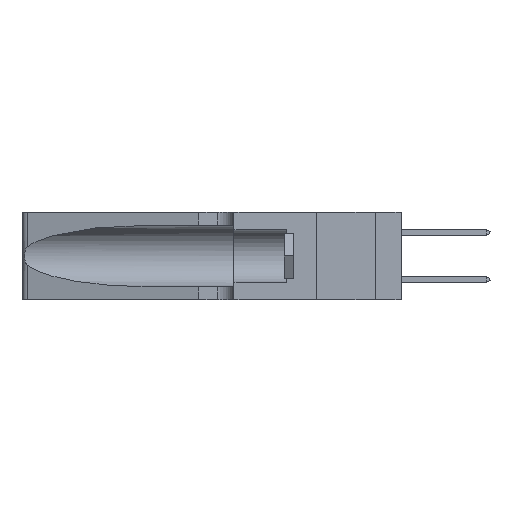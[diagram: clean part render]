
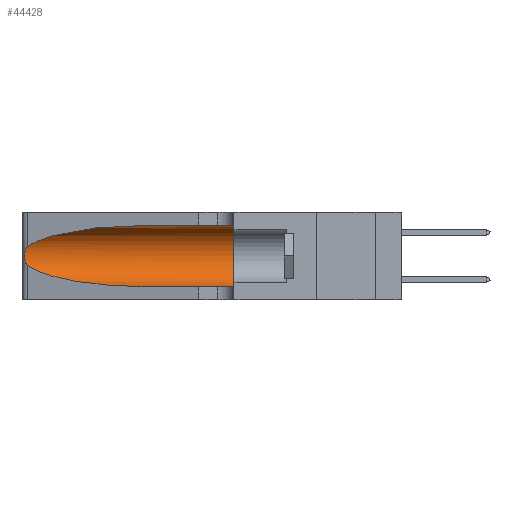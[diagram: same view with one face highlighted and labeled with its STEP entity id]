
A CAD part, left-side view. The second image highlights one B-rep face of the part: STEP entity #44428.
In plain terms, the highlighted cylindrical face has radius 3.308 mm (diameter 6.617 mm), a partial arc.
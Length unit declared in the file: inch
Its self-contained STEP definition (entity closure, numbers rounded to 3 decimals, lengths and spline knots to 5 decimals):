
#996 = CARTESIAN_POINT ( 'NONE',  ( 0.25487, 1.22718, 0.14631 ) ) ;
#1841 = VERTEX_POINT ( 'NONE', #12380 ) ;
#2195 = EDGE_CURVE ( 'NONE', #1841, #40838, #9917, .T. ) ;
#2207 = CARTESIAN_POINT ( 'NONE',  ( 0.25487, 1.22718, 0.22369 ) ) ;
#2439 = DIRECTION ( 'NONE',  ( 0., -1., 0. ) ) ;
#2642 = EDGE_CURVE ( 'NONE', #31339, #1841, #34223, .T. ) ;
#3109 = CARTESIAN_POINT ( 'NONE',  ( 0.1305, 1.61858, 0.31525 ) ) ;
#4090 = CARTESIAN_POINT ( 'NONE',  ( 0.1305, 0.35, 0.185 ) ) ;
#4380 = CARTESIAN_POINT ( 'NONE',  ( 0.25787, 1.23484, 0.2124 ) ) ;
#7574 = CARTESIAN_POINT ( 'NONE',  ( 0.26018, 1.23835, 0.19895 ) ) ;
#9135 = EDGE_CURVE ( 'NONE', #31339, #39985, #35731, .T. ) ;
#9268 = CARTESIAN_POINT ( 'NONE',  ( 0.1305, 1.61858, 0.05475 ) ) ;
#9917 = CIRCLE ( 'NONE', #42887, 0.13025 ) ;
#10337 = ORIENTED_EDGE ( 'NONE', *, *, #40380, .T. ) ;
#11255 = DIRECTION ( 'NONE',  ( 0., 1., 0. ) ) ;
#11530 = FACE_OUTER_BOUND ( 'NONE', #39396, .T. ) ;
#11571 = CARTESIAN_POINT ( 'NONE',  ( 0.25639, 1.23186, 0.15144 ) ) ;
#11637 = VERTEX_POINT ( 'NONE', #42432 ) ;
#12380 = CARTESIAN_POINT ( 'NONE',  ( 0.1305, 0.35, 0.31525 ) ) ;
#13915 = DIRECTION ( 'NONE',  ( 0., 0., -1. ) ) ;
#14069 = VECTOR ( 'NONE', #2439, 39.37008 ) ;
#14387 = CYLINDRICAL_SURFACE ( 'NONE', #37112, 0.13025 ) ;
#14938 = CARTESIAN_POINT ( 'NONE',  ( 0.25487, 1.22718, 0.22369 ) ) ;
#15084 = CARTESIAN_POINT ( 'NONE',  ( 0.25789, 1.23486, 0.15765 ) ) ;
#16788 = CARTESIAN_POINT ( 'NONE',  ( 0.18966, 0.96281, 0.05475 ) ) ;
#17612 = DIRECTION ( 'NONE',  ( 0., -1., 0. ) ) ;
#18283 = CARTESIAN_POINT ( 'NONE',  ( 0.18966, 0.96281, 0.31525 ) ) ;
#18475 = CARTESIAN_POINT ( 'NONE',  ( 0.26075, 1.23896, 0.178 ) ) ;
#18594 = ORIENTED_EDGE ( 'NONE', *, *, #41261, .T. ) ;
#19185 = EDGE_CURVE ( 'NONE', #11637, #39734, #34885, .T. ) ;
#20119 = ORIENTED_EDGE ( 'NONE', *, *, #2642, .F. ) ;
#22096 = CARTESIAN_POINT ( 'NONE',  ( 0.25555, 1.22993, 0.14849 ) ) ;
#22246 = CARTESIAN_POINT ( 'NONE',  ( 0.25639, 1.23184, 0.21858 ) ) ;
#22397 = CARTESIAN_POINT ( 'NONE',  ( 0.25555, 1.22994, 0.2215 ) ) ;
#22699 = CARTESIAN_POINT ( 'NONE',  ( 0.26075, 1.23896, 0.19203 ) ) ;
#23720 = LINE ( 'NONE', #9268, #14069 ) ;
#25239 = CARTESIAN_POINT ( 'NONE',  ( 0.1305, 0.72297, 0.31525 ) ) ;
#25550 = CARTESIAN_POINT ( 'NONE',  ( 0.25487, 1.22718, 0.22369 ) ) ;
#26036 = CARTESIAN_POINT ( 'NONE',  ( 0.25487, 1.22718, 0.14631 ) ) ;
#26040 = DIRECTION ( 'NONE',  ( 0., 0., 1. ) ) ;
#26438 = CARTESIAN_POINT ( 'NONE',  ( 0.2373, 1.15595, 0.08982 ) ) ;
#28228 = ORIENTED_EDGE ( 'NONE', *, *, #2195, .F. ) ;
#30805 = CARTESIAN_POINT ( 'NONE',  ( 0.1305, 0.72297, 0.05475 ) ) ;
#31339 = VERTEX_POINT ( 'NONE', #35454 ) ;
#31789 = CARTESIAN_POINT ( 'NONE',  ( 0.1305, 0.35, 0.05475 ) ) ;
#33256 = CARTESIAN_POINT ( 'NONE',  ( 0.26017, 1.23833, 0.17102 ) ) ;
#34223 = LINE ( 'NONE', #3109, #42796 ) ;
#34885 =( BOUNDED_CURVE ( )  B_SPLINE_CURVE ( 3, ( #996, #26438, #16788, #30805 ),
 .UNSPECIFIED., .F., .T. ) 
 B_SPLINE_CURVE_WITH_KNOTS ( ( 4, 4 ),
 ( 3.44316, 4.71239 ),
 .UNSPECIFIED. ) 
 CURVE ( )  GEOMETRIC_REPRESENTATION_ITEM ( )  RATIONAL_B_SPLINE_CURVE ( ( 1., 0.87, 0.87, 1. ) ) 
 REPRESENTATION_ITEM ( '' )  );
#35209 = ORIENTED_EDGE ( 'NONE', *, *, #19185, .T. ) ;
#35454 = CARTESIAN_POINT ( 'NONE',  ( 0.1305, 0.72297, 0.31525 ) ) ;
#35731 =( BOUNDED_CURVE ( )  B_SPLINE_CURVE ( 3, ( #25239, #18283, #43603, #25550 ),
 .UNSPECIFIED., .F., .F. ) 
 B_SPLINE_CURVE_WITH_KNOTS ( ( 4, 4 ),
 ( 1.5708, 2.84003 ),
 .UNSPECIFIED. ) 
 CURVE ( )  GEOMETRIC_REPRESENTATION_ITEM ( )  RATIONAL_B_SPLINE_CURVE ( ( 1., 0.87, 0.87, 1. ) ) 
 REPRESENTATION_ITEM ( '' )  );
#37112 = AXIS2_PLACEMENT_3D ( 'NONE', #42608, #46564, #13915 ) ;
#39396 = EDGE_LOOP ( 'NONE', ( #39607, #10337, #35209, #18594, #28228, #20119 ) ) ;
#39607 = ORIENTED_EDGE ( 'NONE', *, *, #9135, .T. ) ;
#39734 = VERTEX_POINT ( 'NONE', #44288 ) ;
#39985 = VERTEX_POINT ( 'NONE', #2207 ) ;
#40263 = CARTESIAN_POINT ( 'NONE',  ( 0.25854, 1.2359, 0.20912 ) ) ;
#40380 = EDGE_CURVE ( 'NONE', #39985, #11637, #42755, .T. ) ;
#40838 = VERTEX_POINT ( 'NONE', #31789 ) ;
#41261 = EDGE_CURVE ( 'NONE', #39734, #40838, #23720, .T. ) ;
#42432 = CARTESIAN_POINT ( 'NONE',  ( 0.25487, 1.22718, 0.14631 ) ) ;
#42608 = CARTESIAN_POINT ( 'NONE',  ( 0.1305, 1.61858, 0.185 ) ) ;
#42755 = B_SPLINE_CURVE_WITH_KNOTS ( 'NONE', 3,
 ( #14938, #22397, #22246, #4380, #40263, #7574, #22699, #18475, #33256, #43783, #15084, #11571, #22096, #26036 ),
 .UNSPECIFIED., .F., .F.,
 ( 4, 2, 2, 2, 2, 2, 4 ),
 ( 0., 0.00027, 0.00053, 0.00107, 0.0016, 0.00187, 0.00214 ),
 .UNSPECIFIED. ) ;
#42796 = VECTOR ( 'NONE', #17612, 39.37008 ) ;
#42887 = AXIS2_PLACEMENT_3D ( 'NONE', #4090, #11255, #26040 ) ;
#43603 = CARTESIAN_POINT ( 'NONE',  ( 0.2373, 1.15595, 0.28018 ) ) ;
#43783 = CARTESIAN_POINT ( 'NONE',  ( 0.25856, 1.23593, 0.16098 ) ) ;
#44288 = CARTESIAN_POINT ( 'NONE',  ( 0.1305, 0.72297, 0.05475 ) ) ;
#44428 = ADVANCED_FACE ( 'NONE', ( #11530 ), #14387, .F. ) ;
#46564 = DIRECTION ( 'NONE',  ( 0., -1., 0. ) ) ;
